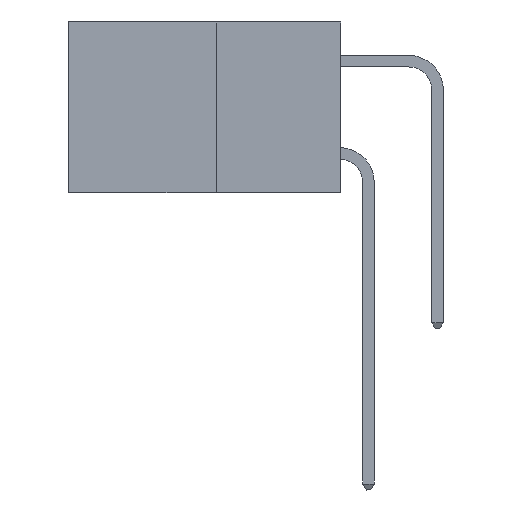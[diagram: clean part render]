
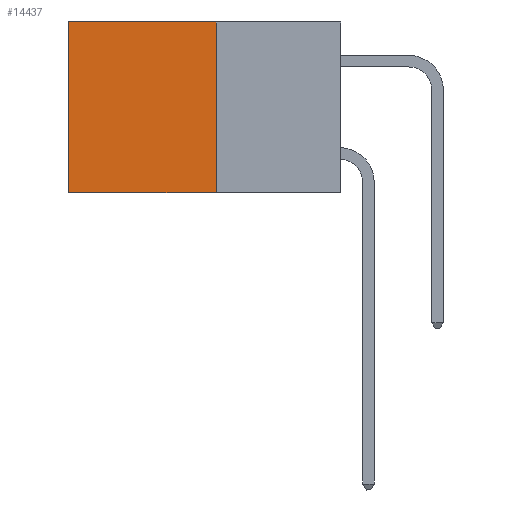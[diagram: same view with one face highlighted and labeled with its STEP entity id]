
A CAD part, left-side view. The second image highlights one B-rep face of the part: STEP entity #14437.
In plain terms, the highlighted planar face has unit normal (-1, 0, 0).
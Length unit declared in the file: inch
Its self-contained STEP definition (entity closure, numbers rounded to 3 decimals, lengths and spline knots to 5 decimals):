
#286 = CARTESIAN_POINT ( 'NONE',  ( 0.277, 0.27, -0.37 ) ) ;
#933 = DIRECTION ( 'NONE',  ( 0., 0., -1. ) ) ;
#1067 = CARTESIAN_POINT ( 'NONE',  ( 0.277, 0.59, -0.37 ) ) ;
#1073 = AXIS2_PLACEMENT_3D ( 'NONE', #15805, #17233, #8667 ) ;
#1905 = CARTESIAN_POINT ( 'NONE',  ( 0.277, 0.27, 0. ) ) ;
#1917 = LINE ( 'NONE', #1067, #16467 ) ;
#2236 = EDGE_CURVE ( 'NONE', #10821, #4486, #10187, .T. ) ;
#2799 = VERTEX_POINT ( 'NONE', #10845 ) ;
#3007 = ORIENTED_EDGE ( 'NONE', *, *, #13266, .F. ) ;
#3352 = VECTOR ( 'NONE', #10253, 39.37008 ) ;
#3652 = EDGE_LOOP ( 'NONE', ( #9255, #5890, #3007, #11499 ) ) ;
#4486 = VERTEX_POINT ( 'NONE', #17066 ) ;
#4660 = DIRECTION ( 'NONE',  ( 0., 0., -1. ) ) ;
#5653 = LINE ( 'NONE', #6007, #16612 ) ;
#5890 = ORIENTED_EDGE ( 'NONE', *, *, #12480, .F. ) ;
#6007 = CARTESIAN_POINT ( 'NONE',  ( 0.277, 0.27, -0.37 ) ) ;
#6235 = LINE ( 'NONE', #286, #3352 ) ;
#6382 = VECTOR ( 'NONE', #7187, 39.37008 ) ;
#7187 = DIRECTION ( 'NONE',  ( 0., 1., 0. ) ) ;
#7223 = PLANE ( 'NONE',  #1073 ) ;
#8524 = EDGE_CURVE ( 'NONE', #4486, #2799, #1917, .T. ) ;
#8667 = DIRECTION ( 'NONE',  ( 0., 0., -1. ) ) ;
#8756 = CARTESIAN_POINT ( 'NONE',  ( 0.277, 0.27, -0.37 ) ) ;
#9255 = ORIENTED_EDGE ( 'NONE', *, *, #8524, .T. ) ;
#10187 = LINE ( 'NONE', #1905, #6382 ) ;
#10253 = DIRECTION ( 'NONE',  ( 0., 1., 0. ) ) ;
#10821 = VERTEX_POINT ( 'NONE', #14939 ) ;
#10845 = CARTESIAN_POINT ( 'NONE',  ( 0.277, 0.59, -0.37 ) ) ;
#11499 = ORIENTED_EDGE ( 'NONE', *, *, #2236, .T. ) ;
#12480 = EDGE_CURVE ( 'NONE', #16732, #2799, #6235, .T. ) ;
#12787 = FACE_OUTER_BOUND ( 'NONE', #3652, .T. ) ;
#13266 = EDGE_CURVE ( 'NONE', #10821, #16732, #5653, .T. ) ;
#14437 = ADVANCED_FACE ( 'NONE', ( #12787 ), #7223, .F. ) ;
#14939 = CARTESIAN_POINT ( 'NONE',  ( 0.277, 0.27, 0. ) ) ;
#15805 = CARTESIAN_POINT ( 'NONE',  ( 0.277, 0.27, -0.37 ) ) ;
#16467 = VECTOR ( 'NONE', #933, 39.37008 ) ;
#16612 = VECTOR ( 'NONE', #4660, 39.37008 ) ;
#16732 = VERTEX_POINT ( 'NONE', #8756 ) ;
#17066 = CARTESIAN_POINT ( 'NONE',  ( 0.277, 0.59, 0. ) ) ;
#17233 = DIRECTION ( 'NONE',  ( 1., 0., 0. ) ) ;
